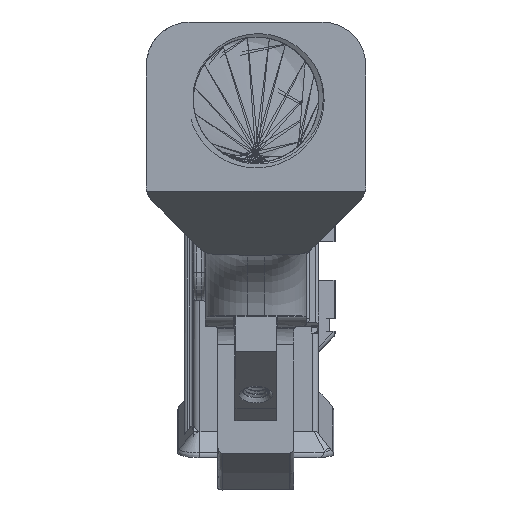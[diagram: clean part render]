
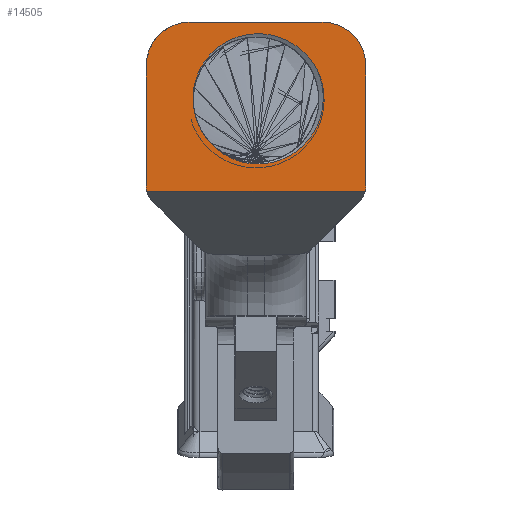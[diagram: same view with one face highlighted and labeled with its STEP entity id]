
A CAD part, front view. The second image highlights one B-rep face of the part: STEP entity #14505.
In plain terms, the highlighted planar face has unit normal (0, -1, 0).
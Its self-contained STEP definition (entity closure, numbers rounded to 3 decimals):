
#273=FACE_BOUND('',#2305,.T.);
#510=PLANE('',#15787);
#1483=FACE_OUTER_BOUND('',#2304,.T.);
#2304=EDGE_LOOP('',(#13405,#13406,#13407,#13408,#13409,#13410,#13411,#13412));
#2305=EDGE_LOOP('',(#13413,#13414,#13415));
#2306=CIRCLE('',#14521,14.288);
#2730=CIRCLE('',#15673,5.);
#2737=CIRCLE('',#15695,10.);
#2752=CIRCLE('',#15780,10.);
#2753=CIRCLE('',#15783,5.);
#3402=B_SPLINE_CURVE_WITH_KNOTS('',3,(#67584,#67585,#67586,#67587,#67588,
#67589,#67590,#67591,#67592,#67593,#67594,#67595,#67596,#67597,#67598,#67599,
#67600,#67601,#67602,#67603),.UNSPECIFIED.,.F.,.F.,(4,2,2,2,2,2,2,2,2,4),
(-5.554,-5.144,-4.751,-3.987,
-3.1,-2.295,-1.558,-0.888,
-0.276,0.),.UNSPECIFIED.);
#3454=B_SPLINE_CURVE_WITH_KNOTS('',3,(#79730,#79731,#79732,#79733,#79734,
#79735,#79736,#79737,#79738,#79739,#79740,#79741,#79742,#79743,#79744,#79745,
#79746,#79747),.UNSPECIFIED.,.F.,.F.,(4,2,2,2,2,2,2,2,4),(-3.265,
-3.064,-2.805,-2.391,-1.927,-1.429,
-0.873,-0.576,0.),.UNSPECIFIED.);
#4308=LINE('',#70422,#5198);
#4310=LINE('',#70427,#5200);
#4342=LINE('',#78999,#5232);
#4344=LINE('',#79006,#5234);
#5198=VECTOR('',#18989,10.);
#5200=VECTOR('',#18993,10.);
#5232=VECTOR('',#19201,10.);
#5234=VECTOR('',#19211,10.);
#5237=VERTEX_POINT('',#19221);
#5238=VERTEX_POINT('',#19234);
#6633=VERTEX_POINT('',#67583);
#6634=VERTEX_POINT('',#68861);
#6635=VERTEX_POINT('',#68862);
#6642=VERTEX_POINT('',#70421);
#6643=VERTEX_POINT('',#70425);
#6644=VERTEX_POINT('',#70426);
#6699=VERTEX_POINT('',#78994);
#6700=VERTEX_POINT('',#78998);
#6701=VERTEX_POINT('',#79002);
#6704=EDGE_CURVE('',#5238,#5237,#2306,.T.);
#8791=EDGE_CURVE('',#6633,#5238,#3402,.T.);
#8795=EDGE_CURVE('',#6634,#6635,#2730,.T.);
#8813=EDGE_CURVE('',#6635,#6642,#4308,.T.);
#8815=EDGE_CURVE('',#6643,#6644,#4310,.T.);
#8818=EDGE_CURVE('',#6642,#6643,#2737,.T.);
#8932=EDGE_CURVE('',#6644,#6699,#2752,.T.);
#8934=EDGE_CURVE('',#6699,#6700,#4342,.T.);
#8936=EDGE_CURVE('',#6700,#6701,#2753,.T.);
#8938=EDGE_CURVE('',#6701,#6634,#4344,.T.);
#8939=EDGE_CURVE('',#5237,#6633,#3454,.T.);
#13405=ORIENTED_EDGE('',*,*,#8932,.T.);
#13406=ORIENTED_EDGE('',*,*,#8934,.T.);
#13407=ORIENTED_EDGE('',*,*,#8936,.T.);
#13408=ORIENTED_EDGE('',*,*,#8938,.T.);
#13409=ORIENTED_EDGE('',*,*,#8795,.T.);
#13410=ORIENTED_EDGE('',*,*,#8813,.T.);
#13411=ORIENTED_EDGE('',*,*,#8818,.T.);
#13412=ORIENTED_EDGE('',*,*,#8815,.T.);
#13413=ORIENTED_EDGE('',*,*,#6704,.T.);
#13414=ORIENTED_EDGE('',*,*,#8939,.T.);
#13415=ORIENTED_EDGE('',*,*,#8791,.T.);
#14505=ADVANCED_FACE('',(#1483,#273),#510,.T.);
#14521=AXIS2_PLACEMENT_3D('',#19235,#15793,#15794);
#15673=AXIS2_PLACEMENT_3D('',#68863,#18941,#18942);
#15695=AXIS2_PLACEMENT_3D('',#70431,#18998,#18999);
#15780=AXIS2_PLACEMENT_3D('',#78995,#19196,#19197);
#15783=AXIS2_PLACEMENT_3D('',#79003,#19205,#19206);
#15787=AXIS2_PLACEMENT_3D('',#79748,#19214,#19215);
#15793=DIRECTION('center_axis',(0.,1.,
0.));
#15794=DIRECTION('ref_axis',(0.,0.,
-1.));
#18941=DIRECTION('center_axis',(0.,-1.,
0.));
#18942=DIRECTION('ref_axis',(0.,0.,1.));
#18989=DIRECTION('',(0.,0.,1.));
#18993=DIRECTION('',(-1.,0.,0.));
#18998=DIRECTION('center_axis',(0.,-1.,
0.));
#18999=DIRECTION('ref_axis',(0.,0.,1.));
#19196=DIRECTION('center_axis',(0.,-1.,
0.));
#19197=DIRECTION('ref_axis',(0.,0.,1.));
#19201=DIRECTION('',(0.,0.,-1.));
#19205=DIRECTION('center_axis',(0.,-1.,
0.));
#19206=DIRECTION('ref_axis',(0.,0.,
-1.));
#19211=DIRECTION('',(1.,0.,-0.001));
#19214=DIRECTION('center_axis',(0.,-1.,
0.));
#19215=DIRECTION('ref_axis',(0.,0.,-1.));
#19221=CARTESIAN_POINT('',(8.079,-128.574,36.347));
#19234=CARTESIAN_POINT('',(12.585,-128.572,27.008));
#19235=CARTESIAN_POINT('Origin',(22.323,-128.567,37.463));
#67583=CARTESIAN_POINT('',(36.257,-128.561,44.265));
#67584=CARTESIAN_POINT('Ctrl Pts',(36.257,-128.561,44.265));
#67585=CARTESIAN_POINT('Ctrl Pts',(36.603,-128.561,43.504));
#67586=CARTESIAN_POINT('Ctrl Pts',(36.89,-128.561,42.712));
#67587=CARTESIAN_POINT('Ctrl Pts',(37.319,-128.561,41.12));
#67588=CARTESIAN_POINT('Ctrl Pts',(37.468,-128.561,40.325));
#67589=CARTESIAN_POINT('Ctrl Pts',(37.718,-128.561,37.962));
#67590=CARTESIAN_POINT('Ctrl Pts',(37.642,-128.561,36.384));
#67591=CARTESIAN_POINT('Ctrl Pts',(36.961,-128.561,33.06));
#67592=CARTESIAN_POINT('Ctrl Pts',(36.241,-128.561,31.17));
#67593=CARTESIAN_POINT('Ctrl Pts',(33.946,-128.562,27.778));
#67594=CARTESIAN_POINT('Ctrl Pts',(32.55,-128.563,26.393));
#67595=CARTESIAN_POINT('Ctrl Pts',(29.443,-128.564,24.329));
#67596=CARTESIAN_POINT('Ctrl Pts',(27.644,-128.565,23.517));
#67597=CARTESIAN_POINT('Ctrl Pts',(23.72,-128.567,22.746));
#67598=CARTESIAN_POINT('Ctrl Pts',(21.797,-128.568,22.748));
#67599=CARTESIAN_POINT('Ctrl Pts',(18.222,-128.569,23.458));
#67600=CARTESIAN_POINT('Ctrl Pts',(16.419,-128.57,24.133));
#67601=CARTESIAN_POINT('Ctrl Pts',(13.955,-128.571,25.775));
#67602=CARTESIAN_POINT('Ctrl Pts',(13.239,-128.571,26.359));
#67603=CARTESIAN_POINT('Ctrl Pts',(12.585,-128.572,27.008));
#68861=CARTESIAN_POINT('',(47.173,-128.557,16.655));
#68862=CARTESIAN_POINT('',(47.322,-128.556,17.87));
#68863=CARTESIAN_POINT('Origin',(42.322,-128.559,17.87));
#70421=CARTESIAN_POINT('',(47.324,-128.556,45.165));
#70422=CARTESIAN_POINT('',(47.322,-128.556,4.9));
#70425=CARTESIAN_POINT('',(37.324,-128.561,55.166));
#70426=CARTESIAN_POINT('',(7.324,-128.574,55.167));
#70427=CARTESIAN_POINT('',(34.843,-128.562,55.166));
#70431=CARTESIAN_POINT('Origin',(37.324,-128.561,45.166));
#78994=CARTESIAN_POINT('',(-2.676,-128.578,45.168));
#78995=CARTESIAN_POINT('Origin',(7.324,-128.574,45.167));
#78998=CARTESIAN_POINT('',(-2.678,-128.578,17.872));
#78999=CARTESIAN_POINT('',(-2.678,-128.578,4.902));
#79002=CARTESIAN_POINT('',(-2.535,-128.578,16.686));
#79003=CARTESIAN_POINT('Origin',(2.322,-128.576,17.872));
#79006=CARTESIAN_POINT('',(17.255,-128.57,16.674));
#79730=CARTESIAN_POINT('Ctrl Pts',(8.079,-128.574,36.347));
#79731=CARTESIAN_POINT('Ctrl Pts',(7.917,-128.574,37.823));
#79732=CARTESIAN_POINT('Ctrl Pts',(7.985,-128.574,39.315));
#79733=CARTESIAN_POINT('Ctrl Pts',(8.662,-128.573,42.643));
#79734=CARTESIAN_POINT('Ctrl Pts',(9.347,-128.573,44.105));
#79735=CARTESIAN_POINT('Ctrl Pts',(10.887,-128.572,46.769));
#79736=CARTESIAN_POINT('Ctrl Pts',(12.144,-128.572,48.209));
#79737=CARTESIAN_POINT('Ctrl Pts',(15.317,-128.57,50.674));
#79738=CARTESIAN_POINT('Ctrl Pts',(17.131,-128.57,51.499));
#79739=CARTESIAN_POINT('Ctrl Pts',(20.753,-128.568,52.472));
#79740=CARTESIAN_POINT('Ctrl Pts',(22.705,-128.567,52.608));
#79741=CARTESIAN_POINT('Ctrl Pts',(26.782,-128.565,52.1));
#79742=CARTESIAN_POINT('Ctrl Pts',(28.693,-128.565,51.388));
#79743=CARTESIAN_POINT('Ctrl Pts',(31.16,-128.564,49.971));
#79744=CARTESIAN_POINT('Ctrl Pts',(31.97,-128.563,49.394));
#79745=CARTESIAN_POINT('Ctrl Pts',(34.168,-128.562,47.485));
#79746=CARTESIAN_POINT('Ctrl Pts',(35.368,-128.562,45.966));
#79747=CARTESIAN_POINT('Ctrl Pts',(36.257,-128.561,44.265));
#79748=CARTESIAN_POINT('Origin',(22.36,-128.567,1.735));
